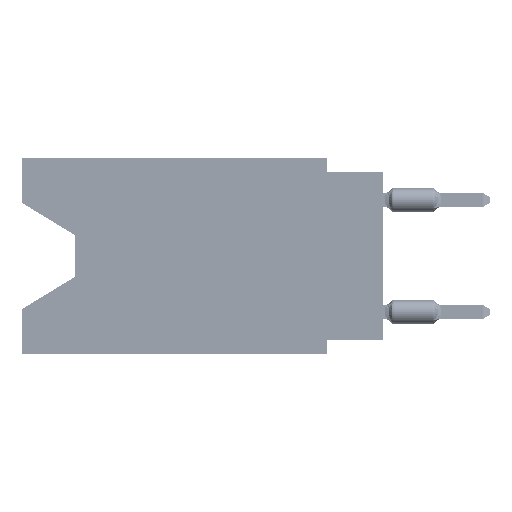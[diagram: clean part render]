
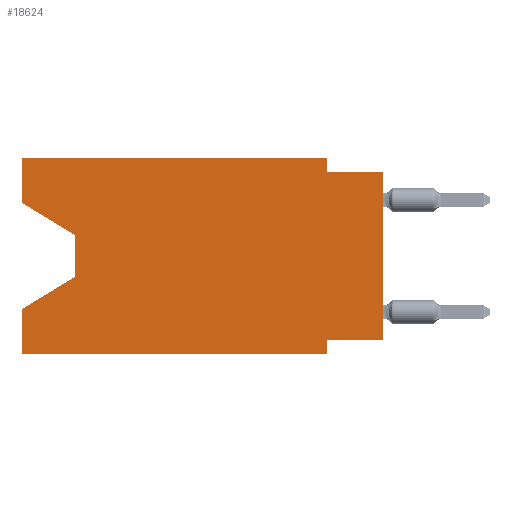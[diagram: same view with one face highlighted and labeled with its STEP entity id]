
A CAD part, left-side view. The second image highlights one B-rep face of the part: STEP entity #18624.
In plain terms, the highlighted planar face has unit normal (-1, 0, 0).
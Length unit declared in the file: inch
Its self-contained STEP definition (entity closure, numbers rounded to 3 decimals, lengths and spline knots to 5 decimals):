
#2204 = VERTEX_POINT ( 'NONE', #65134 ) ;
#4776 = ORIENTED_EDGE ( 'NONE', *, *, #15653, .T. ) ;
#6268 = DIRECTION ( 'NONE',  ( 0., -1., 0. ) ) ;
#10161 = ORIENTED_EDGE ( 'NONE', *, *, #14968, .F. ) ;
#10393 = LINE ( 'NONE', #79283, #40810 ) ;
#12020 = VERTEX_POINT ( 'NONE', #51662 ) ;
#14420 = CARTESIAN_POINT ( 'NONE',  ( 0., 0.645, 0. ) ) ;
#14785 = CARTESIAN_POINT ( 'NONE',  ( 0., 0., -0.025 ) ) ;
#14885 = LINE ( 'NONE', #31431, #50836 ) ;
#14968 = EDGE_CURVE ( 'NONE', #80068, #100897, #57493, .T. ) ;
#15653 = EDGE_CURVE ( 'NONE', #2204, #109398, #62428, .T. ) ;
#16559 = EDGE_CURVE ( 'NONE', #52341, #100897, #69447, .T. ) ;
#16699 = CARTESIAN_POINT ( 'NONE',  ( 0., 0.55, -0.212 ) ) ;
#17657 = DIRECTION ( 'NONE',  ( 0., -1., 0. ) ) ;
#18624 = ADVANCED_FACE ( 'NONE', ( #51560 ), #76605, .F. ) ;
#19829 = EDGE_CURVE ( 'NONE', #59093, #73961, #53265, .T. ) ;
#20698 = ORIENTED_EDGE ( 'NONE', *, *, #16559, .T. ) ;
#22979 = LINE ( 'NONE', #14420, #67875 ) ;
#26210 = CARTESIAN_POINT ( 'NONE',  ( 0., 0.645, -0.35 ) ) ;
#26868 = ORIENTED_EDGE ( 'NONE', *, *, #39224, .T. ) ;
#26997 = VERTEX_POINT ( 'NONE', #104974 ) ;
#28053 = VECTOR ( 'NONE', #33793, 39.37008 ) ;
#28162 = EDGE_CURVE ( 'NONE', #26997, #73961, #92768, .T. ) ;
#29336 = CARTESIAN_POINT ( 'NONE',  ( 0., 0.1, -0.325 ) ) ;
#29981 = CARTESIAN_POINT ( 'NONE',  ( 0., 0.1, -0.35 ) ) ;
#31431 = CARTESIAN_POINT ( 'NONE',  ( 0., 0.645, 0. ) ) ;
#31586 = ORIENTED_EDGE ( 'NONE', *, *, #52514, .F. ) ;
#33225 = CARTESIAN_POINT ( 'NONE',  ( 0., 0., -0.325 ) ) ;
#33548 = CARTESIAN_POINT ( 'NONE',  ( 0., 0., -0.325 ) ) ;
#33793 = DIRECTION ( 'NONE',  ( 0., 1., 0. ) ) ;
#39224 = EDGE_CURVE ( 'NONE', #109398, #77575, #87315, .T. ) ;
#40439 = DIRECTION ( 'NONE',  ( 0., 0., -1. ) ) ;
#40810 = VECTOR ( 'NONE', #90998, 39.37008 ) ;
#41759 = LINE ( 'NONE', #57150, #56558 ) ;
#42482 = DIRECTION ( 'NONE',  ( 0., 0., 1. ) ) ;
#43512 = DIRECTION ( 'NONE',  ( 0., 0., -1. ) ) ;
#43564 = CARTESIAN_POINT ( 'NONE',  ( 0., 0.55, -0.138 ) ) ;
#43679 = DIRECTION ( 'NONE',  ( 0., -0.855, -0.519 ) ) ;
#43852 = ORIENTED_EDGE ( 'NONE', *, *, #28162, .F. ) ;
#44129 = EDGE_CURVE ( 'NONE', #59093, #80068, #92980, .T. ) ;
#45208 = VERTEX_POINT ( 'NONE', #79438 ) ;
#49459 = CARTESIAN_POINT ( 'NONE',  ( 0., 0., -0.025 ) ) ;
#50836 = VECTOR ( 'NONE', #108822, 39.37008 ) ;
#50992 = CARTESIAN_POINT ( 'NONE',  ( 0., 0.645, 0. ) ) ;
#51560 = FACE_OUTER_BOUND ( 'NONE', #52535, .T. ) ;
#51662 = CARTESIAN_POINT ( 'NONE',  ( 0., 0.645, -0.26975 ) ) ;
#52341 = VERTEX_POINT ( 'NONE', #82654 ) ;
#52514 = EDGE_CURVE ( 'NONE', #110196, #45208, #14885, .T. ) ;
#52535 = EDGE_LOOP ( 'NONE', ( #4776, #26868, #57375, #105679, #20698, #10161, #98564, #71790, #43852, #107341, #31586, #74978 ) ) ;
#53265 = LINE ( 'NONE', #69209, #64430 ) ;
#56558 = VECTOR ( 'NONE', #75346, 39.37008 ) ;
#57150 = CARTESIAN_POINT ( 'NONE',  ( 0., 0.1, 0. ) ) ;
#57375 = ORIENTED_EDGE ( 'NONE', *, *, #88678, .T. ) ;
#57493 = LINE ( 'NONE', #64380, #103915 ) ;
#59093 = VERTEX_POINT ( 'NONE', #33548 ) ;
#59998 = CARTESIAN_POINT ( 'NONE',  ( 0., 0.55, -0.138 ) ) ;
#60367 = VECTOR ( 'NONE', #43679, 39.37008 ) ;
#62428 = LINE ( 'NONE', #97159, #60367 ) ;
#64380 = CARTESIAN_POINT ( 'NONE',  ( 0., 0.1, -0.35 ) ) ;
#64430 = VECTOR ( 'NONE', #42482, 39.37008 ) ;
#65134 = CARTESIAN_POINT ( 'NONE',  ( 0., 0.645, -0.08025 ) ) ;
#67875 = VECTOR ( 'NONE', #76434, 39.37008 ) ;
#69209 = CARTESIAN_POINT ( 'NONE',  ( 0., 0., 0. ) ) ;
#69447 = LINE ( 'NONE', #26210, #89360 ) ;
#71790 = ORIENTED_EDGE ( 'NONE', *, *, #19829, .T. ) ;
#73961 = VERTEX_POINT ( 'NONE', #49459 ) ;
#74978 = ORIENTED_EDGE ( 'NONE', *, *, #92253, .F. ) ;
#75346 = DIRECTION ( 'NONE',  ( 0., 0., -1. ) ) ;
#76434 = DIRECTION ( 'NONE',  ( 0., 0., 1. ) ) ;
#76605 = PLANE ( 'NONE',  #86035 ) ;
#77575 = VERTEX_POINT ( 'NONE', #103912 ) ;
#78302 = DIRECTION ( 'NONE',  ( 1., 0., 0. ) ) ;
#79283 = CARTESIAN_POINT ( 'NONE',  ( 0., 0.645, 0. ) ) ;
#79438 = CARTESIAN_POINT ( 'NONE',  ( 0., 0.1, 0. ) ) ;
#80068 = VERTEX_POINT ( 'NONE', #29336 ) ;
#82654 = CARTESIAN_POINT ( 'NONE',  ( 0., 0.645, -0.35 ) ) ;
#83841 = VECTOR ( 'NONE', #6268, 39.37008 ) ;
#86035 = AXIS2_PLACEMENT_3D ( 'NONE', #50992, #78302, #105047 ) ;
#87315 = LINE ( 'NONE', #59998, #94948 ) ;
#88678 = EDGE_CURVE ( 'NONE', #77575, #12020, #102649, .T. ) ;
#89360 = VECTOR ( 'NONE', #17657, 39.37008 ) ;
#89409 = VECTOR ( 'NONE', #93554, 39.37008 ) ;
#90998 = DIRECTION ( 'NONE',  ( 0., 0., 1. ) ) ;
#92253 = EDGE_CURVE ( 'NONE', #2204, #110196, #22979, .T. ) ;
#92768 = LINE ( 'NONE', #14785, #83841 ) ;
#92980 = LINE ( 'NONE', #33225, #28053 ) ;
#93554 = DIRECTION ( 'NONE',  ( 0., 0.855, -0.519 ) ) ;
#94948 = VECTOR ( 'NONE', #43512, 39.37008 ) ;
#97159 = CARTESIAN_POINT ( 'NONE',  ( 0., 0.645, -0.08025 ) ) ;
#98564 = ORIENTED_EDGE ( 'NONE', *, *, #44129, .F. ) ;
#100897 = VERTEX_POINT ( 'NONE', #29981 ) ;
#102649 = LINE ( 'NONE', #16699, #89409 ) ;
#102742 = EDGE_CURVE ( 'NONE', #45208, #26997, #41759, .T. ) ;
#103912 = CARTESIAN_POINT ( 'NONE',  ( 0., 0.55, -0.212 ) ) ;
#103915 = VECTOR ( 'NONE', #40439, 39.37008 ) ;
#104974 = CARTESIAN_POINT ( 'NONE',  ( 0., 0.1, -0.025 ) ) ;
#105047 = DIRECTION ( 'NONE',  ( 0., 0., -1. ) ) ;
#105679 = ORIENTED_EDGE ( 'NONE', *, *, #106487, .F. ) ;
#106487 = EDGE_CURVE ( 'NONE', #52341, #12020, #10393, .T. ) ;
#107341 = ORIENTED_EDGE ( 'NONE', *, *, #102742, .F. ) ;
#108822 = DIRECTION ( 'NONE',  ( 0., -1., 0. ) ) ;
#109398 = VERTEX_POINT ( 'NONE', #43564 ) ;
#110196 = VERTEX_POINT ( 'NONE', #112162 ) ;
#112162 = CARTESIAN_POINT ( 'NONE',  ( 0., 0.645, 0. ) ) ;
